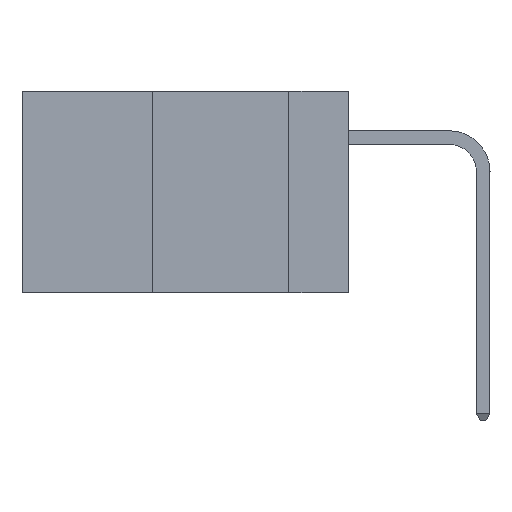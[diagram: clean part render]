
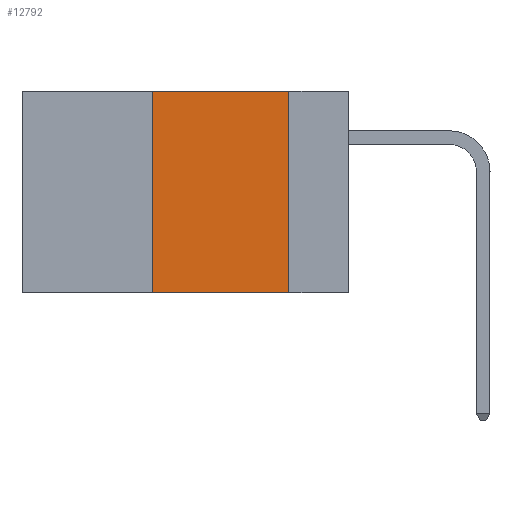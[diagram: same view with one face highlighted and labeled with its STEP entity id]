
A CAD part, left-side view. The second image highlights one B-rep face of the part: STEP entity #12792.
In plain terms, the highlighted planar face has unit normal (-1, 0, 0).
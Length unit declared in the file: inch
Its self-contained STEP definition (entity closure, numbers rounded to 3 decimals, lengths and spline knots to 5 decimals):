
#1755 = DIRECTION ( 'NONE',  ( 0., 0., -1. ) ) ;
#2303 = VERTEX_POINT ( 'NONE', #9646 ) ;
#2498 = EDGE_CURVE ( 'NONE', #10820, #2303, #7717, .T. ) ;
#2562 = ORIENTED_EDGE ( 'NONE', *, *, #8333, .T. ) ;
#3040 = ORIENTED_EDGE ( 'NONE', *, *, #2498, .F. ) ;
#3117 = LINE ( 'NONE', #4841, #14374 ) ;
#3319 = DIRECTION ( 'NONE',  ( 0., 0., 1. ) ) ;
#3388 = DIRECTION ( 'NONE',  ( 0., -1., 0. ) ) ;
#4754 = CARTESIAN_POINT ( 'NONE',  ( 0., 0.36, -0.37 ) ) ;
#4841 = CARTESIAN_POINT ( 'NONE',  ( 0., 0.11, 0. ) ) ;
#5165 = CARTESIAN_POINT ( 'NONE',  ( 0., 0.36, 0. ) ) ;
#5554 = VECTOR ( 'NONE', #12173, 39.37008 ) ;
#5660 = DIRECTION ( 'NONE',  ( 0., 0., -1. ) ) ;
#5803 = EDGE_CURVE ( 'NONE', #2303, #13302, #3117, .T. ) ;
#6262 = CARTESIAN_POINT ( 'NONE',  ( 0., 0.36, 0. ) ) ;
#6351 = FACE_OUTER_BOUND ( 'NONE', #15642, .T. ) ;
#6494 = VERTEX_POINT ( 'NONE', #4754 ) ;
#6527 = EDGE_CURVE ( 'NONE', #6494, #10820, #10804, .T. ) ;
#7256 = AXIS2_PLACEMENT_3D ( 'NONE', #13017, #14427, #5660 ) ;
#7717 = LINE ( 'NONE', #8679, #18629 ) ;
#8333 = EDGE_CURVE ( 'NONE', #6494, #13302, #17104, .T. ) ;
#8679 = CARTESIAN_POINT ( 'NONE',  ( 0., 0.6, 0. ) ) ;
#9646 = CARTESIAN_POINT ( 'NONE',  ( 0., 0.11, 0. ) ) ;
#10706 = CARTESIAN_POINT ( 'NONE',  ( 0., 0.6, -0.37 ) ) ;
#10804 = LINE ( 'NONE', #6262, #17832 ) ;
#10820 = VERTEX_POINT ( 'NONE', #5165 ) ;
#11612 = PLANE ( 'NONE',  #7256 ) ;
#12173 = DIRECTION ( 'NONE',  ( 0., -1., 0. ) ) ;
#12792 = ADVANCED_FACE ( 'NONE', ( #6351 ), #11612, .F. ) ;
#13017 = CARTESIAN_POINT ( 'NONE',  ( 0., 0.6, 0. ) ) ;
#13302 = VERTEX_POINT ( 'NONE', #17099 ) ;
#14303 = ORIENTED_EDGE ( 'NONE', *, *, #6527, .F. ) ;
#14374 = VECTOR ( 'NONE', #1755, 39.37008 ) ;
#14427 = DIRECTION ( 'NONE',  ( 1., 0., 0. ) ) ;
#14759 = ORIENTED_EDGE ( 'NONE', *, *, #5803, .F. ) ;
#15642 = EDGE_LOOP ( 'NONE', ( #14759, #3040, #14303, #2562 ) ) ;
#17099 = CARTESIAN_POINT ( 'NONE',  ( 0., 0.11, -0.37 ) ) ;
#17104 = LINE ( 'NONE', #10706, #5554 ) ;
#17832 = VECTOR ( 'NONE', #3319, 39.37008 ) ;
#18629 = VECTOR ( 'NONE', #3388, 39.37008 ) ;
